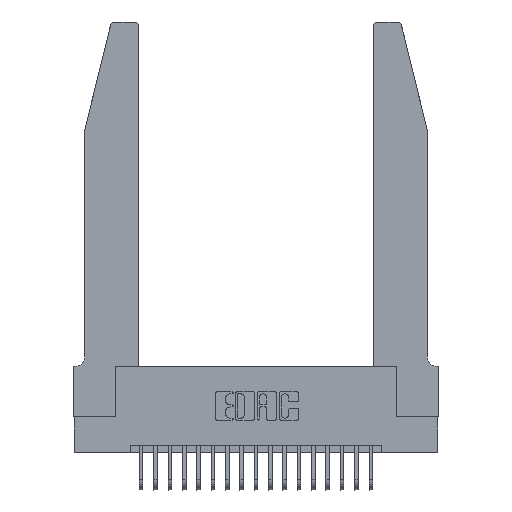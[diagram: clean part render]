
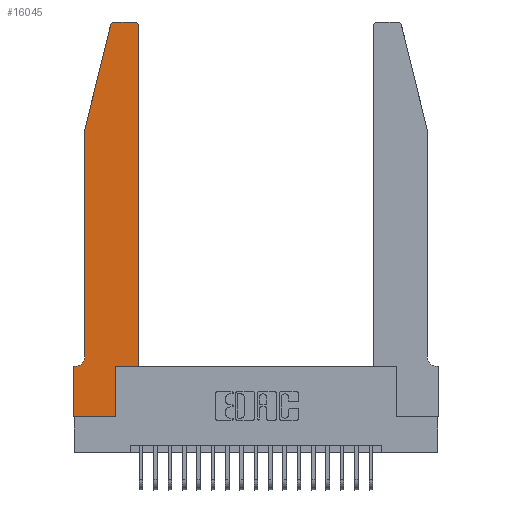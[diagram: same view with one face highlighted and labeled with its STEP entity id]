
A CAD part, top view. The second image highlights one B-rep face of the part: STEP entity #16045.
In plain terms, the highlighted planar face has unit normal (0, 0, 1).
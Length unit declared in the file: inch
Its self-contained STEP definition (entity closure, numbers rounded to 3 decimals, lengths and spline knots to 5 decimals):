
#113 = VERTEX_POINT ( 'NONE', #15771 ) ;
#402 = CIRCLE ( 'NONE', #10313, 0.03 ) ;
#645 = ORIENTED_EDGE ( 'NONE', *, *, #11927, .T. ) ;
#680 = CARTESIAN_POINT ( 'NONE',  ( 0.4505, 0.35, 0.37 ) ) ;
#706 = AXIS2_PLACEMENT_3D ( 'NONE', #11226, #12839, #3045 ) ;
#898 = VECTOR ( 'NONE', #15803, 39.37008 ) ;
#1015 = ORIENTED_EDGE ( 'NONE', *, *, #5856, .T. ) ;
#1098 = CARTESIAN_POINT ( 'NONE',  ( 0.0055, 0.42, 0.37 ) ) ;
#1156 = CARTESIAN_POINT ( 'NONE',  ( 0.0755, 0.35, 0.37 ) ) ;
#1157 = VECTOR ( 'NONE', #8328, 39.37008 ) ;
#1225 = LINE ( 'NONE', #680, #13772 ) ;
#1261 = CARTESIAN_POINT ( 'NONE',  ( 0.0755, 0.42, 0.37 ) ) ;
#1412 = CIRCLE ( 'NONE', #19135, 0.07 ) ;
#1630 = CARTESIAN_POINT ( 'NONE',  ( 0.25487, 2.72718, 0.37 ) ) ;
#2068 = DIRECTION ( 'NONE',  ( 1., 0., 0. ) ) ;
#2238 = EDGE_CURVE ( 'NONE', #16509, #11449, #18731, .T. ) ;
#2658 = CARTESIAN_POINT ( 'NONE',  ( 0.0755, 2., 0.37 ) ) ;
#2801 = DIRECTION ( 'NONE',  ( -1., 0., 0. ) ) ;
#2809 = LINE ( 'NONE', #13512, #6700 ) ;
#3045 = DIRECTION ( 'NONE',  ( 1., 0., 0. ) ) ;
#3069 = VECTOR ( 'NONE', #3639, 39.37008 ) ;
#3138 = EDGE_CURVE ( 'NONE', #7096, #16509, #10723, .T. ) ;
#3263 = VERTEX_POINT ( 'NONE', #1630 ) ;
#3639 = DIRECTION ( 'NONE',  ( -1., 0., 0. ) ) ;
#3678 = EDGE_CURVE ( 'NONE', #18562, #18919, #7925, .T. ) ;
#3834 = CARTESIAN_POINT ( 'NONE',  ( 0., 0., 0.37 ) ) ;
#4058 = CARTESIAN_POINT ( 'NONE',  ( 0.0055, 0.35, 0.37 ) ) ;
#4416 = LINE ( 'NONE', #2658, #16770 ) ;
#4548 = CARTESIAN_POINT ( 'NONE',  ( 0.4505, 0.35, 0.37 ) ) ;
#4765 = DIRECTION ( 'NONE',  ( 0., 0., 1. ) ) ;
#5181 = VECTOR ( 'NONE', #19267, 39.37008 ) ;
#5349 = FACE_OUTER_BOUND ( 'NONE', #7217, .T. ) ;
#5686 = EDGE_CURVE ( 'NONE', #3263, #20139, #4416, .T. ) ;
#5831 = CARTESIAN_POINT ( 'NONE',  ( 0.0755, 2., 0.37 ) ) ;
#5856 = EDGE_CURVE ( 'NONE', #10958, #16164, #18028, .T. ) ;
#6317 = VECTOR ( 'NONE', #7855, 39.37008 ) ;
#6431 = CARTESIAN_POINT ( 'NONE',  ( 0.2865, 0.35, 0.37 ) ) ;
#6527 = CARTESIAN_POINT ( 'NONE',  ( 0., 0., 0.37 ) ) ;
#6700 = VECTOR ( 'NONE', #2068, 39.37008 ) ;
#6921 = ORIENTED_EDGE ( 'NONE', *, *, #3678, .T. ) ;
#7096 = VERTEX_POINT ( 'NONE', #19902 ) ;
#7217 = EDGE_LOOP ( 'NONE', ( #16884, #19133, #9472, #14957, #645, #6921, #7475, #20521, #1015, #7347, #17123, #9200 ) ) ;
#7347 = ORIENTED_EDGE ( 'NONE', *, *, #12782, .T. ) ;
#7475 = ORIENTED_EDGE ( 'NONE', *, *, #8150, .T. ) ;
#7855 = DIRECTION ( 'NONE',  ( 1., 0., 0. ) ) ;
#7925 = LINE ( 'NONE', #1156, #898 ) ;
#8150 = EDGE_CURVE ( 'NONE', #18919, #11694, #14714, .T. ) ;
#8242 = CARTESIAN_POINT ( 'NONE',  ( 0.2865, 0., 0.37 ) ) ;
#8328 = DIRECTION ( 'NONE',  ( 0., -1., 0. ) ) ;
#8522 = CARTESIAN_POINT ( 'NONE',  ( 0.284, 2.72, 0.37 ) ) ;
#8587 = VERTEX_POINT ( 'NONE', #1261 ) ;
#8610 = CARTESIAN_POINT ( 'NONE',  ( 0.2605, 2.75, 0.37 ) ) ;
#8901 = VECTOR ( 'NONE', #18684, 39.37008 ) ;
#9200 = ORIENTED_EDGE ( 'NONE', *, *, #3138, .T. ) ;
#9472 = ORIENTED_EDGE ( 'NONE', *, *, #5686, .T. ) ;
#10133 = DIRECTION ( 'NONE',  ( 1., 0., 0. ) ) ;
#10313 = AXIS2_PLACEMENT_3D ( 'NONE', #8522, #19710, #10133 ) ;
#10639 = LINE ( 'NONE', #4548, #6317 ) ;
#10723 = CIRCLE ( 'NONE', #13097, 0.03 ) ;
#10839 = DIRECTION ( 'NONE',  ( -0.239, -0.971, 0. ) ) ;
#10958 = VERTEX_POINT ( 'NONE', #8242 ) ;
#11084 = EDGE_CURVE ( 'NONE', #11449, #3263, #402, .T. ) ;
#11226 = CARTESIAN_POINT ( 'NONE',  ( 0., 0.35, 0.37 ) ) ;
#11449 = VERTEX_POINT ( 'NONE', #20952 ) ;
#11569 = CARTESIAN_POINT ( 'NONE',  ( 0., 0.35, 0.37 ) ) ;
#11694 = VERTEX_POINT ( 'NONE', #3834 ) ;
#11927 = EDGE_CURVE ( 'NONE', #8587, #18562, #1412, .T. ) ;
#12597 = DIRECTION ( 'NONE',  ( 0., 0., -1. ) ) ;
#12782 = EDGE_CURVE ( 'NONE', #16164, #113, #10639, .T. ) ;
#12839 = DIRECTION ( 'NONE',  ( 0., 0., 1. ) ) ;
#13097 = AXIS2_PLACEMENT_3D ( 'NONE', #14476, #4765, #16039 ) ;
#13194 = LINE ( 'NONE', #5831, #8901 ) ;
#13512 = CARTESIAN_POINT ( 'NONE',  ( 0., 0., 0.37 ) ) ;
#13772 = VECTOR ( 'NONE', #16887, 39.37008 ) ;
#14196 = CARTESIAN_POINT ( 'NONE',  ( 0.4205, 2.75, 0.37 ) ) ;
#14476 = CARTESIAN_POINT ( 'NONE',  ( 0.4205, 2.72, 0.37 ) ) ;
#14714 = LINE ( 'NONE', #6527, #1157 ) ;
#14912 = EDGE_CURVE ( 'NONE', #11694, #10958, #2809, .T. ) ;
#14957 = ORIENTED_EDGE ( 'NONE', *, *, #19910, .T. ) ;
#15771 = CARTESIAN_POINT ( 'NONE',  ( 0.4505, 0.35, 0.37 ) ) ;
#15803 = DIRECTION ( 'NONE',  ( -1., 0., 0. ) ) ;
#16039 = DIRECTION ( 'NONE',  ( 1., 0., 0. ) ) ;
#16045 = ADVANCED_FACE ( 'NONE', ( #5349 ), #20754, .T. ) ;
#16164 = VERTEX_POINT ( 'NONE', #17961 ) ;
#16509 = VERTEX_POINT ( 'NONE', #14196 ) ;
#16770 = VECTOR ( 'NONE', #10839, 39.37008 ) ;
#16884 = ORIENTED_EDGE ( 'NONE', *, *, #2238, .T. ) ;
#16887 = DIRECTION ( 'NONE',  ( 0., 1., 0. ) ) ;
#17123 = ORIENTED_EDGE ( 'NONE', *, *, #17576, .T. ) ;
#17576 = EDGE_CURVE ( 'NONE', #113, #7096, #1225, .T. ) ;
#17961 = CARTESIAN_POINT ( 'NONE',  ( 0.2865, 0.35, 0.37 ) ) ;
#18028 = LINE ( 'NONE', #6431, #5181 ) ;
#18562 = VERTEX_POINT ( 'NONE', #4058 ) ;
#18684 = DIRECTION ( 'NONE',  ( 0., -1., 0. ) ) ;
#18731 = LINE ( 'NONE', #8610, #3069 ) ;
#18919 = VERTEX_POINT ( 'NONE', #11569 ) ;
#19133 = ORIENTED_EDGE ( 'NONE', *, *, #11084, .T. ) ;
#19135 = AXIS2_PLACEMENT_3D ( 'NONE', #1098, #12597, #2801 ) ;
#19253 = CARTESIAN_POINT ( 'NONE',  ( 0.0755, 2., 0.37 ) ) ;
#19267 = DIRECTION ( 'NONE',  ( 0., 1., 0. ) ) ;
#19710 = DIRECTION ( 'NONE',  ( 0., 0., 1. ) ) ;
#19902 = CARTESIAN_POINT ( 'NONE',  ( 0.4505, 2.72, 0.37 ) ) ;
#19910 = EDGE_CURVE ( 'NONE', #20139, #8587, #13194, .T. ) ;
#20139 = VERTEX_POINT ( 'NONE', #19253 ) ;
#20521 = ORIENTED_EDGE ( 'NONE', *, *, #14912, .T. ) ;
#20754 = PLANE ( 'NONE',  #706 ) ;
#20952 = CARTESIAN_POINT ( 'NONE',  ( 0.284, 2.75, 0.37 ) ) ;
